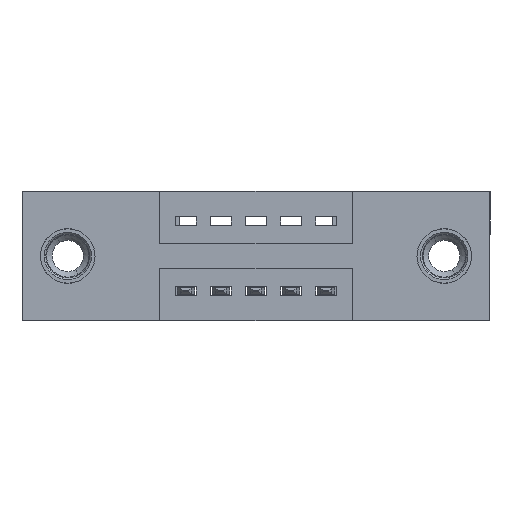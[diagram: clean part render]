
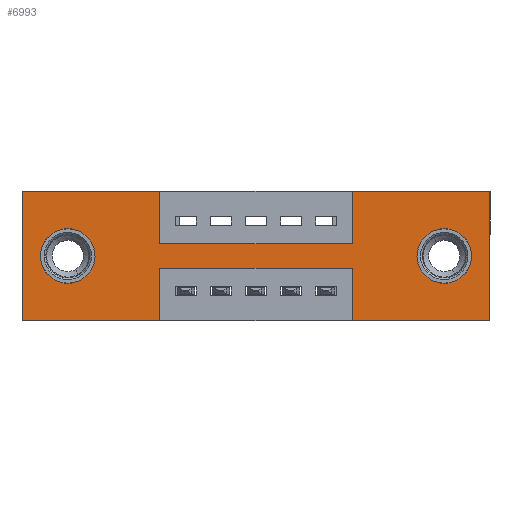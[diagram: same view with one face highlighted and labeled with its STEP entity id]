
A CAD part, front view. The second image highlights one B-rep face of the part: STEP entity #6993.
In plain terms, the highlighted planar face has unit normal (0, -1, 0).
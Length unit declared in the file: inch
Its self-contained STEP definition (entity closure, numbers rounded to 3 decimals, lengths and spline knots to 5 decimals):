
#158 = EDGE_CURVE ( 'NONE', #10007, #3085, #6091, .T. ) ;
#289 = VECTOR ( 'NONE', #970, 39.37008 ) ;
#323 = DIRECTION ( 'NONE',  ( 0., 1., 0. ) ) ;
#544 = LINE ( 'NONE', #9878, #8285 ) ;
#636 = ORIENTED_EDGE ( 'NONE', *, *, #3314, .F. ) ;
#970 = DIRECTION ( 'NONE',  ( 0., 0., 1. ) ) ;
#1011 = PLANE ( 'NONE',  #9473 ) ;
#1125 = LINE ( 'NONE', #2202, #7656 ) ;
#1217 = VERTEX_POINT ( 'NONE', #5058 ) ;
#1247 = CARTESIAN_POINT ( 'NONE',  ( 1.205, 0., -0.185 ) ) ;
#1276 = VERTEX_POINT ( 'NONE', #1284 ) ;
#1284 = CARTESIAN_POINT ( 'NONE',  ( 0.3925, 0., -0.15 ) ) ;
#1478 = CIRCLE ( 'NONE', #4656, 0.078 ) ;
#1579 = ORIENTED_EDGE ( 'NONE', *, *, #7358, .F. ) ;
#1611 = EDGE_LOOP ( 'NONE', ( #3735, #4272, #5494, #636, #10163, #5939, #9553, #2625, #1579, #6885, #4770, #7603 ) ) ;
#1744 = DIRECTION ( 'NONE',  ( 1., 0., 0. ) ) ;
#1783 = VERTEX_POINT ( 'NONE', #5810 ) ;
#1815 = AXIS2_PLACEMENT_3D ( 'NONE', #2277, #3992, #10674 ) ;
#2035 = LINE ( 'NONE', #9844, #8821 ) ;
#2090 = DIRECTION ( 'NONE',  ( 0., 0., 1. ) ) ;
#2202 = CARTESIAN_POINT ( 'NONE',  ( 0., 0., 0. ) ) ;
#2211 = ORIENTED_EDGE ( 'NONE', *, *, #10481, .T. ) ;
#2277 = CARTESIAN_POINT ( 'NONE',  ( 0.13, 0., -0.185 ) ) ;
#2464 = DIRECTION ( 'NONE',  ( 0., 1., 0. ) ) ;
#2625 = ORIENTED_EDGE ( 'NONE', *, *, #6243, .F. ) ;
#2663 = ORIENTED_EDGE ( 'NONE', *, *, #5538, .T. ) ;
#2689 = EDGE_LOOP ( 'NONE', ( #6191, #2211 ) ) ;
#2781 = CIRCLE ( 'NONE', #5093, 0.078 ) ;
#2788 = VERTEX_POINT ( 'NONE', #5004 ) ;
#2869 = DIRECTION ( 'NONE',  ( 0., 0., -1. ) ) ;
#3009 = CARTESIAN_POINT ( 'NONE',  ( 0.3925, 0., -0.37 ) ) ;
#3075 = VERTEX_POINT ( 'NONE', #9667 ) ;
#3085 = VERTEX_POINT ( 'NONE', #4590 ) ;
#3100 = VERTEX_POINT ( 'NONE', #5328 ) ;
#3101 = CARTESIAN_POINT ( 'NONE',  ( 0.9425, 0., 0. ) ) ;
#3102 = EDGE_CURVE ( 'NONE', #7294, #3100, #3641, .T. ) ;
#3164 = EDGE_CURVE ( 'NONE', #1783, #10007, #2035, .T. ) ;
#3177 = DIRECTION ( 'NONE',  ( 0., 1., 0. ) ) ;
#3183 = LINE ( 'NONE', #7653, #7970 ) ;
#3314 = EDGE_CURVE ( 'NONE', #3100, #1783, #544, .T. ) ;
#3571 = FACE_OUTER_BOUND ( 'NONE', #1611, .T. ) ;
#3624 = CARTESIAN_POINT ( 'NONE',  ( 0., 0., -0.37 ) ) ;
#3641 = LINE ( 'NONE', #3665, #5359 ) ;
#3654 = DIRECTION ( 'NONE',  ( -1., 0., 0. ) ) ;
#3665 = CARTESIAN_POINT ( 'NONE',  ( 1.335, 0., 0. ) ) ;
#3711 = EDGE_LOOP ( 'NONE', ( #8191, #2663 ) ) ;
#3735 = ORIENTED_EDGE ( 'NONE', *, *, #9216, .F. ) ;
#3992 = DIRECTION ( 'NONE',  ( 0., 1., 0. ) ) ;
#4044 = EDGE_CURVE ( 'NONE', #7854, #6059, #4404, .T. ) ;
#4170 = CARTESIAN_POINT ( 'NONE',  ( 0.13, 0., -0.263 ) ) ;
#4266 = EDGE_CURVE ( 'NONE', #3075, #9543, #1478, .T. ) ;
#4272 = ORIENTED_EDGE ( 'NONE', *, *, #158, .F. ) ;
#4404 = LINE ( 'NONE', #7659, #10913 ) ;
#4422 = CARTESIAN_POINT ( 'NONE',  ( 1.205, 0., -0.263 ) ) ;
#4590 = CARTESIAN_POINT ( 'NONE',  ( 0.3925, 0., -0.22 ) ) ;
#4656 = AXIS2_PLACEMENT_3D ( 'NONE', #1247, #323, #6403 ) ;
#4770 = ORIENTED_EDGE ( 'NONE', *, *, #5281, .F. ) ;
#4807 = DIRECTION ( 'NONE',  ( -1., 0., 0. ) ) ;
#4873 = CARTESIAN_POINT ( 'NONE',  ( 0.3925, 0., 0. ) ) ;
#4893 = CARTESIAN_POINT ( 'NONE',  ( 0.9425, 0., -0.22 ) ) ;
#5004 = CARTESIAN_POINT ( 'NONE',  ( 0.3925, 0., 0. ) ) ;
#5058 = CARTESIAN_POINT ( 'NONE',  ( 0.13, 0., -0.107 ) ) ;
#5093 = AXIS2_PLACEMENT_3D ( 'NONE', #5138, #2464, #8407 ) ;
#5138 = CARTESIAN_POINT ( 'NONE',  ( 1.205, 0., -0.185 ) ) ;
#5171 = FACE_BOUND ( 'NONE', #2689, .T. ) ;
#5281 = EDGE_CURVE ( 'NONE', #6059, #10870, #1125, .T. ) ;
#5282 = VECTOR ( 'NONE', #3654, 39.37008 ) ;
#5328 = CARTESIAN_POINT ( 'NONE',  ( 1.335, 0., -0.37 ) ) ;
#5359 = VECTOR ( 'NONE', #7864, 39.37008 ) ;
#5364 = DIRECTION ( 'NONE',  ( 0., -1., 0. ) ) ;
#5471 = CIRCLE ( 'NONE', #1815, 0.078 ) ;
#5494 = ORIENTED_EDGE ( 'NONE', *, *, #3164, .F. ) ;
#5538 = EDGE_CURVE ( 'NONE', #9543, #3075, #2781, .T. ) ;
#5543 = VECTOR ( 'NONE', #6633, 39.37008 ) ;
#5606 = CARTESIAN_POINT ( 'NONE',  ( 0., 0., 0. ) ) ;
#5651 = CARTESIAN_POINT ( 'NONE',  ( 1.335, 0., 0. ) ) ;
#5717 = CARTESIAN_POINT ( 'NONE',  ( 0.3925, 0., -0.37 ) ) ;
#5810 = CARTESIAN_POINT ( 'NONE',  ( 0.9425, 0., -0.37 ) ) ;
#5939 = ORIENTED_EDGE ( 'NONE', *, *, #5980, .F. ) ;
#5980 = EDGE_CURVE ( 'NONE', #6629, #7294, #10082, .T. ) ;
#6059 = VERTEX_POINT ( 'NONE', #10944 ) ;
#6091 = LINE ( 'NONE', #6245, #5282 ) ;
#6191 = ORIENTED_EDGE ( 'NONE', *, *, #10493, .T. ) ;
#6243 = EDGE_CURVE ( 'NONE', #1276, #8083, #3183, .T. ) ;
#6245 = CARTESIAN_POINT ( 'NONE',  ( 0.3925, 0., -0.22 ) ) ;
#6337 = DIRECTION ( 'NONE',  ( 0., 0., -1. ) ) ;
#6403 = DIRECTION ( 'NONE',  ( 0., 0., -1. ) ) ;
#6425 = DIRECTION ( 'NONE',  ( 0., 0., 1. ) ) ;
#6432 = CIRCLE ( 'NONE', #6755, 0.078 ) ;
#6629 = VERTEX_POINT ( 'NONE', #3101 ) ;
#6633 = DIRECTION ( 'NONE',  ( 0., 0., -1. ) ) ;
#6637 = LINE ( 'NONE', #8649, #6911 ) ;
#6755 = AXIS2_PLACEMENT_3D ( 'NONE', #8269, #3177, #6425 ) ;
#6838 = EDGE_CURVE ( 'NONE', #10870, #2788, #6637, .T. ) ;
#6885 = ORIENTED_EDGE ( 'NONE', *, *, #6838, .F. ) ;
#6911 = VECTOR ( 'NONE', #9332, 39.37008 ) ;
#6993 = ADVANCED_FACE ( 'NONE', ( #7431, #5171, #3571 ), #1011, .T. ) ;
#7270 = DIRECTION ( 'NONE',  ( 0., 0., 1. ) ) ;
#7294 = VERTEX_POINT ( 'NONE', #5651 ) ;
#7358 = EDGE_CURVE ( 'NONE', #2788, #1276, #9395, .T. ) ;
#7431 = FACE_BOUND ( 'NONE', #3711, .T. ) ;
#7506 = VECTOR ( 'NONE', #6337, 39.37008 ) ;
#7603 = ORIENTED_EDGE ( 'NONE', *, *, #4044, .F. ) ;
#7653 = CARTESIAN_POINT ( 'NONE',  ( 0.3925, 0., -0.15 ) ) ;
#7656 = VECTOR ( 'NONE', #2090, 39.37008 ) ;
#7659 = CARTESIAN_POINT ( 'NONE',  ( 0., 0., -0.37 ) ) ;
#7846 = VECTOR ( 'NONE', #8070, 39.37008 ) ;
#7854 = VERTEX_POINT ( 'NONE', #5717 ) ;
#7864 = DIRECTION ( 'NONE',  ( 0., 0., -1. ) ) ;
#7970 = VECTOR ( 'NONE', #1744, 39.37008 ) ;
#8070 = DIRECTION ( 'NONE',  ( 1., 0., 0. ) ) ;
#8083 = VERTEX_POINT ( 'NONE', #9821 ) ;
#8191 = ORIENTED_EDGE ( 'NONE', *, *, #4266, .T. ) ;
#8269 = CARTESIAN_POINT ( 'NONE',  ( 0.13, 0., -0.185 ) ) ;
#8285 = VECTOR ( 'NONE', #4807, 39.37008 ) ;
#8407 = DIRECTION ( 'NONE',  ( 0., 0., -1. ) ) ;
#8649 = CARTESIAN_POINT ( 'NONE',  ( 0., 0., 0. ) ) ;
#8821 = VECTOR ( 'NONE', #7270, 39.37008 ) ;
#8835 = LINE ( 'NONE', #10171, #289 ) ;
#8882 = EDGE_CURVE ( 'NONE', #8083, #6629, #8835, .T. ) ;
#9216 = EDGE_CURVE ( 'NONE', #3085, #7854, #9217, .T. ) ;
#9217 = LINE ( 'NONE', #3009, #7506 ) ;
#9332 = DIRECTION ( 'NONE',  ( 1., 0., 0. ) ) ;
#9395 = LINE ( 'NONE', #4873, #5543 ) ;
#9473 = AXIS2_PLACEMENT_3D ( 'NONE', #3624, #5364, #2869 ) ;
#9543 = VERTEX_POINT ( 'NONE', #4422 ) ;
#9553 = ORIENTED_EDGE ( 'NONE', *, *, #8882, .F. ) ;
#9667 = CARTESIAN_POINT ( 'NONE',  ( 1.205, 0., -0.107 ) ) ;
#9821 = CARTESIAN_POINT ( 'NONE',  ( 0.9425, 0., -0.15 ) ) ;
#9844 = CARTESIAN_POINT ( 'NONE',  ( 0.9425, 0., -0.37 ) ) ;
#9878 = CARTESIAN_POINT ( 'NONE',  ( 0., 0., -0.37 ) ) ;
#10007 = VERTEX_POINT ( 'NONE', #4893 ) ;
#10082 = LINE ( 'NONE', #5606, #7846 ) ;
#10163 = ORIENTED_EDGE ( 'NONE', *, *, #3102, .F. ) ;
#10171 = CARTESIAN_POINT ( 'NONE',  ( 0.9425, 0., 0. ) ) ;
#10465 = CARTESIAN_POINT ( 'NONE',  ( 0., 0., 0. ) ) ;
#10481 = EDGE_CURVE ( 'NONE', #10574, #1217, #6432, .T. ) ;
#10493 = EDGE_CURVE ( 'NONE', #1217, #10574, #5471, .T. ) ;
#10574 = VERTEX_POINT ( 'NONE', #4170 ) ;
#10674 = DIRECTION ( 'NONE',  ( 0., 0., 1. ) ) ;
#10870 = VERTEX_POINT ( 'NONE', #10465 ) ;
#10913 = VECTOR ( 'NONE', #10985, 39.37008 ) ;
#10944 = CARTESIAN_POINT ( 'NONE',  ( 0., 0., -0.37 ) ) ;
#10985 = DIRECTION ( 'NONE',  ( -1., 0., 0. ) ) ;
